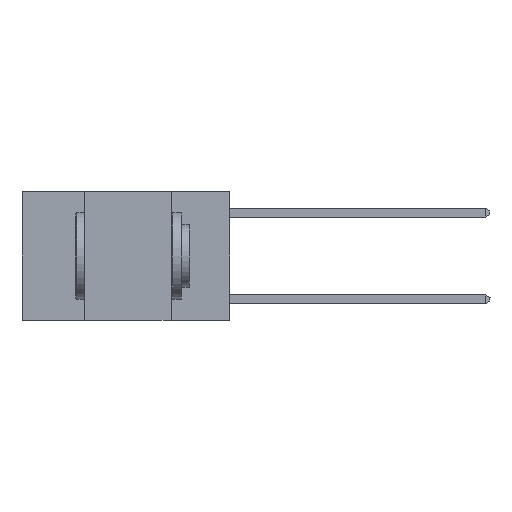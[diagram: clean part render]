
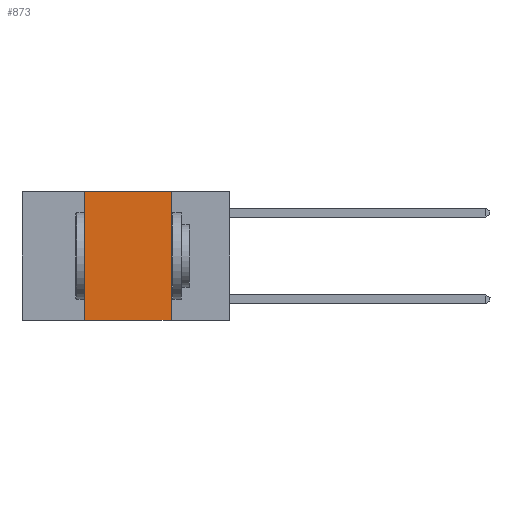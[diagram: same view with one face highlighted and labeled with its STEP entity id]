
A CAD part, left-side view. The second image highlights one B-rep face of the part: STEP entity #873.
In plain terms, the highlighted planar face has unit normal (-1, 0, 0).
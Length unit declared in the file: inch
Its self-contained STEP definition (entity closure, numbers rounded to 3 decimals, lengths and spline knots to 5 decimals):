
#409 = CARTESIAN_POINT ( 'NONE',  ( 0., 0.6, 0. ) ) ;
#612 = VERTEX_POINT ( 'NONE', #31018 ) ;
#873 = ADVANCED_FACE ( 'NONE', ( #20568 ), #14973, .F. ) ;
#1605 = DIRECTION ( 'NONE',  ( 0., 0., 1. ) ) ;
#1658 = DIRECTION ( 'NONE',  ( 0., -1., 0. ) ) ;
#2528 = EDGE_LOOP ( 'NONE', ( #22147, #18486, #17234, #19292 ) ) ;
#2879 = DIRECTION ( 'NONE',  ( 1., 0., 0. ) ) ;
#5267 = VERTEX_POINT ( 'NONE', #19734 ) ;
#5344 = VECTOR ( 'NONE', #26703, 39.37008 ) ;
#6125 = LINE ( 'NONE', #24294, #5344 ) ;
#8110 = EDGE_CURVE ( 'NONE', #612, #10467, #13671, .T. ) ;
#8956 = EDGE_CURVE ( 'NONE', #5267, #612, #14392, .T. ) ;
#9791 = VECTOR ( 'NONE', #1658, 39.37008 ) ;
#10467 = VERTEX_POINT ( 'NONE', #15426 ) ;
#12163 = AXIS2_PLACEMENT_3D ( 'NONE', #409, #2879, #19815 ) ;
#12178 = EDGE_CURVE ( 'NONE', #10467, #23272, #6125, .T. ) ;
#13325 = CARTESIAN_POINT ( 'NONE',  ( 0., 0.6, 0. ) ) ;
#13671 = LINE ( 'NONE', #13325, #19336 ) ;
#14392 = LINE ( 'NONE', #20990, #20769 ) ;
#14973 = PLANE ( 'NONE',  #12163 ) ;
#15426 = CARTESIAN_POINT ( 'NONE',  ( 0., 0.17, 0. ) ) ;
#15778 = DIRECTION ( 'NONE',  ( 0., -1., 0. ) ) ;
#15944 = CARTESIAN_POINT ( 'NONE',  ( 0., 0.17, -0.37 ) ) ;
#16252 = LINE ( 'NONE', #23357, #9791 ) ;
#17066 = EDGE_CURVE ( 'NONE', #5267, #23272, #16252, .T. ) ;
#17234 = ORIENTED_EDGE ( 'NONE', *, *, #8956, .F. ) ;
#18486 = ORIENTED_EDGE ( 'NONE', *, *, #8110, .F. ) ;
#19292 = ORIENTED_EDGE ( 'NONE', *, *, #17066, .T. ) ;
#19336 = VECTOR ( 'NONE', #15778, 39.37008 ) ;
#19734 = CARTESIAN_POINT ( 'NONE',  ( 0., 0.42, -0.37 ) ) ;
#19815 = DIRECTION ( 'NONE',  ( 0., 0., -1. ) ) ;
#20568 = FACE_OUTER_BOUND ( 'NONE', #2528, .T. ) ;
#20769 = VECTOR ( 'NONE', #1605, 39.37008 ) ;
#20990 = CARTESIAN_POINT ( 'NONE',  ( 0., 0.42, 0. ) ) ;
#22147 = ORIENTED_EDGE ( 'NONE', *, *, #12178, .F. ) ;
#23272 = VERTEX_POINT ( 'NONE', #15944 ) ;
#23357 = CARTESIAN_POINT ( 'NONE',  ( 0., 0.6, -0.37 ) ) ;
#24294 = CARTESIAN_POINT ( 'NONE',  ( 0., 0.17, 0. ) ) ;
#26703 = DIRECTION ( 'NONE',  ( 0., 0., -1. ) ) ;
#31018 = CARTESIAN_POINT ( 'NONE',  ( 0., 0.42, 0. ) ) ;
